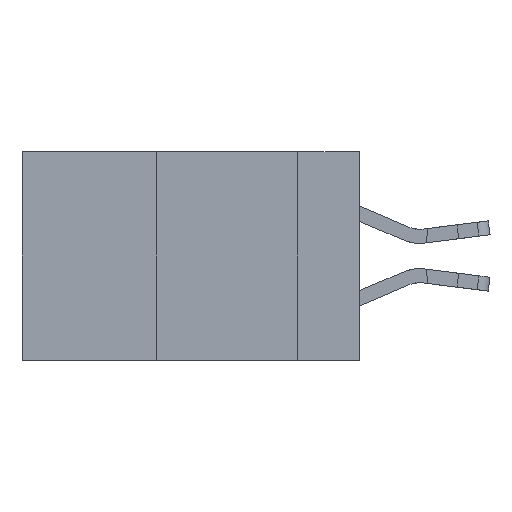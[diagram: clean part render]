
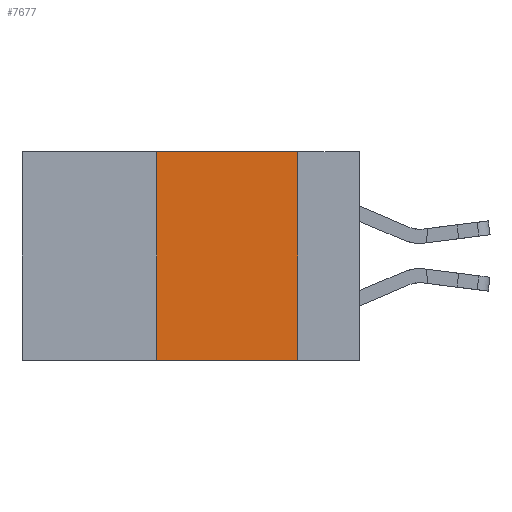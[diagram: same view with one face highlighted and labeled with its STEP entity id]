
A CAD part, left-side view. The second image highlights one B-rep face of the part: STEP entity #7677.
In plain terms, the highlighted planar face has unit normal (-1, 0, 0).
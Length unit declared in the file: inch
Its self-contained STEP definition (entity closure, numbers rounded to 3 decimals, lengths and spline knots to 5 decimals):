
#13 = AXIS2_PLACEMENT_3D ( 'NONE', #22531, #1206, #3057 ) ;
#137 = ORIENTED_EDGE ( 'NONE', *, *, #3802, .F. ) ;
#1206 = DIRECTION ( 'NONE',  ( 1., 0., 0. ) ) ;
#2783 = LINE ( 'NONE', #9830, #18980 ) ;
#3057 = DIRECTION ( 'NONE',  ( 0., 0., -1. ) ) ;
#3089 = CARTESIAN_POINT ( 'NONE',  ( 0., 0.6, 0. ) ) ;
#3802 = EDGE_CURVE ( 'NONE', #14466, #15900, #10354, .T. ) ;
#4002 = LINE ( 'NONE', #3089, #22145 ) ;
#5212 = EDGE_CURVE ( 'NONE', #20338, #6699, #2783, .T. ) ;
#6213 = DIRECTION ( 'NONE',  ( 0., 0., 1. ) ) ;
#6360 = FACE_OUTER_BOUND ( 'NONE', #8338, .T. ) ;
#6699 = VERTEX_POINT ( 'NONE', #6949 ) ;
#6825 = DIRECTION ( 'NONE',  ( 0., 0., -1. ) ) ;
#6949 = CARTESIAN_POINT ( 'NONE',  ( 0., 0.36, 0. ) ) ;
#7677 = ADVANCED_FACE ( 'NONE', ( #6360 ), #13795, .F. ) ;
#8338 = EDGE_LOOP ( 'NONE', ( #137, #11744, #21296, #16103 ) ) ;
#9667 = EDGE_CURVE ( 'NONE', #20338, #15900, #21835, .T. ) ;
#9830 = CARTESIAN_POINT ( 'NONE',  ( 0., 0.36, 0. ) ) ;
#9849 = CARTESIAN_POINT ( 'NONE',  ( 0., 0.6, -0.37 ) ) ;
#9910 = CARTESIAN_POINT ( 'NONE',  ( 0., 0.11, -0.37 ) ) ;
#10354 = LINE ( 'NONE', #13923, #13109 ) ;
#11515 = CARTESIAN_POINT ( 'NONE',  ( 0., 0.36, -0.37 ) ) ;
#11744 = ORIENTED_EDGE ( 'NONE', *, *, #13523, .F. ) ;
#12227 = DIRECTION ( 'NONE',  ( 0., -1., 0. ) ) ;
#13109 = VECTOR ( 'NONE', #6825, 39.37008 ) ;
#13523 = EDGE_CURVE ( 'NONE', #6699, #14466, #4002, .T. ) ;
#13795 = PLANE ( 'NONE',  #13 ) ;
#13923 = CARTESIAN_POINT ( 'NONE',  ( 0., 0.11, 0. ) ) ;
#14466 = VERTEX_POINT ( 'NONE', #20258 ) ;
#15613 = DIRECTION ( 'NONE',  ( 0., -1., 0. ) ) ;
#15900 = VERTEX_POINT ( 'NONE', #9910 ) ;
#16103 = ORIENTED_EDGE ( 'NONE', *, *, #9667, .T. ) ;
#18980 = VECTOR ( 'NONE', #6213, 39.37008 ) ;
#20258 = CARTESIAN_POINT ( 'NONE',  ( 0., 0.11, 0. ) ) ;
#20338 = VERTEX_POINT ( 'NONE', #11515 ) ;
#21296 = ORIENTED_EDGE ( 'NONE', *, *, #5212, .F. ) ;
#21835 = LINE ( 'NONE', #9849, #22401 ) ;
#22145 = VECTOR ( 'NONE', #15613, 39.37008 ) ;
#22401 = VECTOR ( 'NONE', #12227, 39.37008 ) ;
#22531 = CARTESIAN_POINT ( 'NONE',  ( 0., 0.6, 0. ) ) ;
